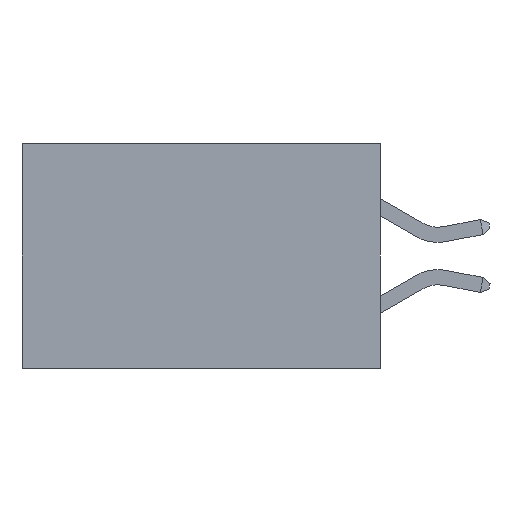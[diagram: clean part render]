
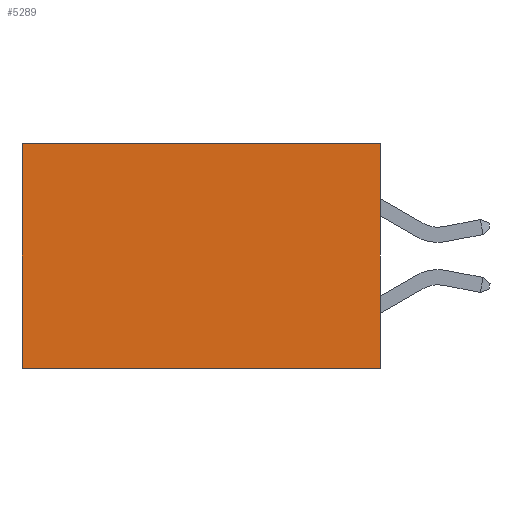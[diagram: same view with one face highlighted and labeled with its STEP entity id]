
A CAD part, left-side view. The second image highlights one B-rep face of the part: STEP entity #5289.
In plain terms, the highlighted planar face has unit normal (-1, 0, 0).
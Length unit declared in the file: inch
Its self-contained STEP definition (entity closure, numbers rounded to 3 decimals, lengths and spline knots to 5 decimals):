
#205 = CARTESIAN_POINT ( 'NONE',  ( 0.277, 0., 0. ) ) ;
#364 = FACE_OUTER_BOUND ( 'NONE', #1225, .T. ) ;
#517 = VECTOR ( 'NONE', #5992, 39.37008 ) ;
#999 = VERTEX_POINT ( 'NONE', #7715 ) ;
#1089 = ORIENTED_EDGE ( 'NONE', *, *, #5329, .F. ) ;
#1225 = EDGE_LOOP ( 'NONE', ( #1594, #1089, #3728, #1325 ) ) ;
#1325 = ORIENTED_EDGE ( 'NONE', *, *, #7800, .T. ) ;
#1594 = ORIENTED_EDGE ( 'NONE', *, *, #4279, .T. ) ;
#1823 = LINE ( 'NONE', #3335, #3676 ) ;
#2774 = PLANE ( 'NONE',  #8850 ) ;
#2845 = DIRECTION ( 'NONE',  ( 0., 0., -1. ) ) ;
#2866 = DIRECTION ( 'NONE',  ( 1., 0., 0. ) ) ;
#2883 = CARTESIAN_POINT ( 'NONE',  ( 0.277, 0., -0.37 ) ) ;
#3133 = EDGE_CURVE ( 'NONE', #7953, #5359, #7903, .T. ) ;
#3321 = DIRECTION ( 'NONE',  ( 0., 1., 0. ) ) ;
#3335 = CARTESIAN_POINT ( 'NONE',  ( 0.277, 0., -0.37 ) ) ;
#3676 = VECTOR ( 'NONE', #3321, 39.37008 ) ;
#3728 = ORIENTED_EDGE ( 'NONE', *, *, #3133, .F. ) ;
#3904 = CARTESIAN_POINT ( 'NONE',  ( 0.277, 0., 0. ) ) ;
#4025 = CARTESIAN_POINT ( 'NONE',  ( 0.277, 0., -0.37 ) ) ;
#4246 = VECTOR ( 'NONE', #6214, 39.37008 ) ;
#4279 = EDGE_CURVE ( 'NONE', #999, #6422, #4661, .T. ) ;
#4574 = DIRECTION ( 'NONE',  ( 0., 1., 0. ) ) ;
#4661 = LINE ( 'NONE', #6031, #517 ) ;
#5289 = ADVANCED_FACE ( 'NONE', ( #364 ), #2774, .F. ) ;
#5329 = EDGE_CURVE ( 'NONE', #5359, #6422, #1823, .T. ) ;
#5359 = VERTEX_POINT ( 'NONE', #4025 ) ;
#5544 = VECTOR ( 'NONE', #4574, 39.37008 ) ;
#5749 = CARTESIAN_POINT ( 'NONE',  ( 0.277, 0.59, -0.37 ) ) ;
#5992 = DIRECTION ( 'NONE',  ( 0., 0., -1. ) ) ;
#6031 = CARTESIAN_POINT ( 'NONE',  ( 0.277, 0.59, -0.37 ) ) ;
#6214 = DIRECTION ( 'NONE',  ( 0., 0., -1. ) ) ;
#6422 = VERTEX_POINT ( 'NONE', #5749 ) ;
#6432 = CARTESIAN_POINT ( 'NONE',  ( 0.277, 0., -0.37 ) ) ;
#7318 = LINE ( 'NONE', #3904, #5544 ) ;
#7715 = CARTESIAN_POINT ( 'NONE',  ( 0.277, 0.59, 0. ) ) ;
#7800 = EDGE_CURVE ( 'NONE', #7953, #999, #7318, .T. ) ;
#7903 = LINE ( 'NONE', #6432, #4246 ) ;
#7953 = VERTEX_POINT ( 'NONE', #205 ) ;
#8850 = AXIS2_PLACEMENT_3D ( 'NONE', #2883, #2866, #2845 ) ;
